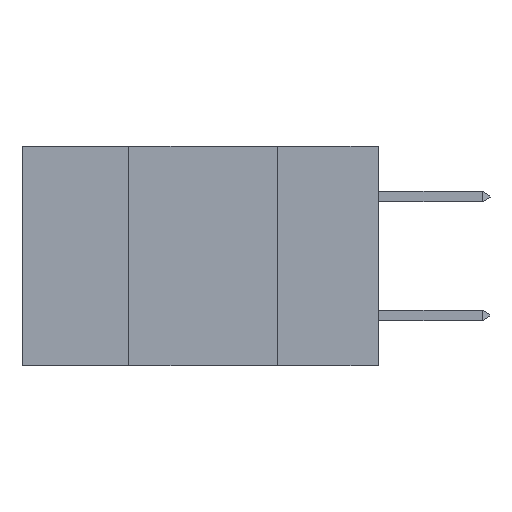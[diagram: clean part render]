
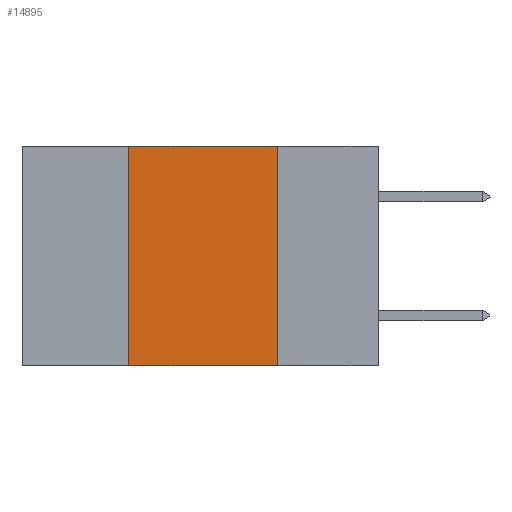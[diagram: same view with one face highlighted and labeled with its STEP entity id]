
A CAD part, left-side view. The second image highlights one B-rep face of the part: STEP entity #14895.
In plain terms, the highlighted planar face has unit normal (-1, 0, 0).
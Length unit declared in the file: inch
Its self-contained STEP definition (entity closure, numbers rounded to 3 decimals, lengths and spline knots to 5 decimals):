
#194 = ORIENTED_EDGE ( 'NONE', *, *, #20084, .F. ) ;
#337 = AXIS2_PLACEMENT_3D ( 'NONE', #14727, #19803, #12992 ) ;
#525 = VERTEX_POINT ( 'NONE', #10875 ) ;
#1095 = CARTESIAN_POINT ( 'NONE',  ( 0., 0.6, 0. ) ) ;
#1307 = ORIENTED_EDGE ( 'NONE', *, *, #14890, .F. ) ;
#1608 = CARTESIAN_POINT ( 'NONE',  ( 0., 0.42, -0.37 ) ) ;
#2820 = PLANE ( 'NONE',  #337 ) ;
#2823 = VECTOR ( 'NONE', #6845, 39.37008 ) ;
#2834 = EDGE_CURVE ( 'NONE', #3206, #525, #12591, .T. ) ;
#3122 = DIRECTION ( 'NONE',  ( 0., -1., 0. ) ) ;
#3206 = VERTEX_POINT ( 'NONE', #1608 ) ;
#3711 = EDGE_CURVE ( 'NONE', #9830, #12677, #11201, .T. ) ;
#4672 = DIRECTION ( 'NONE',  ( 0., 0., 1. ) ) ;
#5020 = VECTOR ( 'NONE', #4672, 39.37008 ) ;
#6429 = ORIENTED_EDGE ( 'NONE', *, *, #2834, .T. ) ;
#6511 = ORIENTED_EDGE ( 'NONE', *, *, #3711, .F. ) ;
#6845 = DIRECTION ( 'NONE',  ( 0., -1., 0. ) ) ;
#9770 = CARTESIAN_POINT ( 'NONE',  ( 0., 0.17, 0. ) ) ;
#9830 = VERTEX_POINT ( 'NONE', #11249 ) ;
#10875 = CARTESIAN_POINT ( 'NONE',  ( 0., 0.17, -0.37 ) ) ;
#11063 = LINE ( 'NONE', #11203, #5020 ) ;
#11201 = LINE ( 'NONE', #1095, #15904 ) ;
#11203 = CARTESIAN_POINT ( 'NONE',  ( 0., 0.42, 0. ) ) ;
#11221 = EDGE_LOOP ( 'NONE', ( #194, #6511, #1307, #6429 ) ) ;
#11249 = CARTESIAN_POINT ( 'NONE',  ( 0., 0.42, 0. ) ) ;
#12591 = LINE ( 'NONE', #18541, #2823 ) ;
#12677 = VERTEX_POINT ( 'NONE', #9770 ) ;
#12992 = DIRECTION ( 'NONE',  ( 0., 0., -1. ) ) ;
#13485 = VECTOR ( 'NONE', #20345, 39.37008 ) ;
#14727 = CARTESIAN_POINT ( 'NONE',  ( 0., 0.6, 0. ) ) ;
#14739 = FACE_OUTER_BOUND ( 'NONE', #11221, .T. ) ;
#14890 = EDGE_CURVE ( 'NONE', #3206, #9830, #11063, .T. ) ;
#14895 = ADVANCED_FACE ( 'NONE', ( #14739 ), #2820, .F. ) ;
#15904 = VECTOR ( 'NONE', #3122, 39.37008 ) ;
#17914 = LINE ( 'NONE', #20264, #13485 ) ;
#18541 = CARTESIAN_POINT ( 'NONE',  ( 0., 0.6, -0.37 ) ) ;
#19803 = DIRECTION ( 'NONE',  ( 1., 0., 0. ) ) ;
#20084 = EDGE_CURVE ( 'NONE', #12677, #525, #17914, .T. ) ;
#20264 = CARTESIAN_POINT ( 'NONE',  ( 0., 0.17, 0. ) ) ;
#20345 = DIRECTION ( 'NONE',  ( 0., 0., -1. ) ) ;
